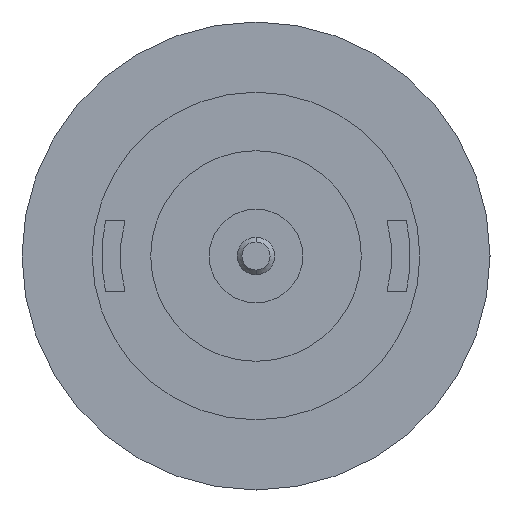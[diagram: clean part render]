
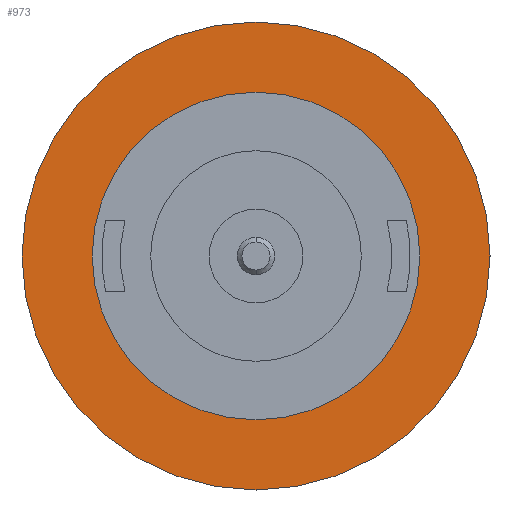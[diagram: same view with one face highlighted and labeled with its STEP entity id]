
A CAD part, front view. The second image highlights one B-rep face of the part: STEP entity #973.
In plain terms, the highlighted planar face has unit normal (0, -1, 0).
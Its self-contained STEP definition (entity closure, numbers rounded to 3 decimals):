
#94 = DIRECTION ( 'NONE',  ( 0., -1., 0. ) ) ;
#174 = DIRECTION ( 'NONE',  ( 0., 0., -1. ) ) ;
#204 = ORIENTED_EDGE ( 'NONE', *, *, #878, .F. ) ;
#231 = CIRCLE ( 'NONE', #1011, 5. ) ;
#268 = EDGE_CURVE ( 'NONE', #358, #584, #1352, .T. ) ;
#316 = DIRECTION ( 'NONE',  ( 0., 0., -1. ) ) ;
#321 = DIRECTION ( 'NONE',  ( 0., -1., 0. ) ) ;
#358 = VERTEX_POINT ( 'NONE', #1357 ) ;
#399 = DIRECTION ( 'NONE',  ( 0., 0., -1. ) ) ;
#422 = DIRECTION ( 'NONE',  ( 0., -1., 0. ) ) ;
#472 = ORIENTED_EDGE ( 'NONE', *, *, #493, .T. ) ;
#493 = EDGE_CURVE ( 'NONE', #1203, #507, #231, .T. ) ;
#499 = ORIENTED_EDGE ( 'NONE', *, *, #724, .T. ) ;
#507 = VERTEX_POINT ( 'NONE', #938 ) ;
#531 = AXIS2_PLACEMENT_3D ( 'NONE', #977, #984, #174 ) ;
#533 = PLANE ( 'NONE',  #1216 ) ;
#539 = DIRECTION ( 'NONE',  ( 0., -1., 0. ) ) ;
#584 = VERTEX_POINT ( 'NONE', #773 ) ;
#618 = AXIS2_PLACEMENT_3D ( 'NONE', #645, #539, #749 ) ;
#645 = CARTESIAN_POINT ( 'NONE',  ( 0., -4.3, 0. ) ) ;
#724 = EDGE_CURVE ( 'NONE', #507, #1203, #1125, .T. ) ;
#743 = DIRECTION ( 'NONE',  ( 0., 0., -1. ) ) ;
#749 = DIRECTION ( 'NONE',  ( 0., 0., -1. ) ) ;
#773 = CARTESIAN_POINT ( 'NONE',  ( 0., -4.3, 3.5 ) ) ;
#821 = CARTESIAN_POINT ( 'NONE',  ( 0., -4.3, 5. ) ) ;
#878 = EDGE_CURVE ( 'NONE', #584, #358, #1103, .T. ) ;
#934 = CARTESIAN_POINT ( 'NONE',  ( 0., -4.3, 0. ) ) ;
#938 = CARTESIAN_POINT ( 'NONE',  ( 0., -4.3, -5. ) ) ;
#949 = EDGE_LOOP ( 'NONE', ( #204, #1233 ) ) ;
#973 = ADVANCED_FACE ( 'NONE', ( #1039, #1067 ), #533, .T. ) ;
#977 = CARTESIAN_POINT ( 'NONE',  ( 0., -4.3, 0. ) ) ;
#984 = DIRECTION ( 'NONE',  ( 0., -1., 0. ) ) ;
#1011 = AXIS2_PLACEMENT_3D ( 'NONE', #1069, #94, #316 ) ;
#1039 = FACE_BOUND ( 'NONE', #949, .T. ) ;
#1067 = FACE_OUTER_BOUND ( 'NONE', #1091, .T. ) ;
#1069 = CARTESIAN_POINT ( 'NONE',  ( 0., -4.3, 0. ) ) ;
#1091 = EDGE_LOOP ( 'NONE', ( #472, #499 ) ) ;
#1103 = CIRCLE ( 'NONE', #618, 3.5 ) ;
#1125 = CIRCLE ( 'NONE', #531, 5. ) ;
#1173 = AXIS2_PLACEMENT_3D ( 'NONE', #934, #422, #399 ) ;
#1203 = VERTEX_POINT ( 'NONE', #821 ) ;
#1216 = AXIS2_PLACEMENT_3D ( 'NONE', #1275, #321, #743 ) ;
#1233 = ORIENTED_EDGE ( 'NONE', *, *, #268, .F. ) ;
#1275 = CARTESIAN_POINT ( 'NONE',  ( 0., -4.3, 0. ) ) ;
#1352 = CIRCLE ( 'NONE', #1173, 3.5 ) ;
#1357 = CARTESIAN_POINT ( 'NONE',  ( 0., -4.3, -3.5 ) ) ;
